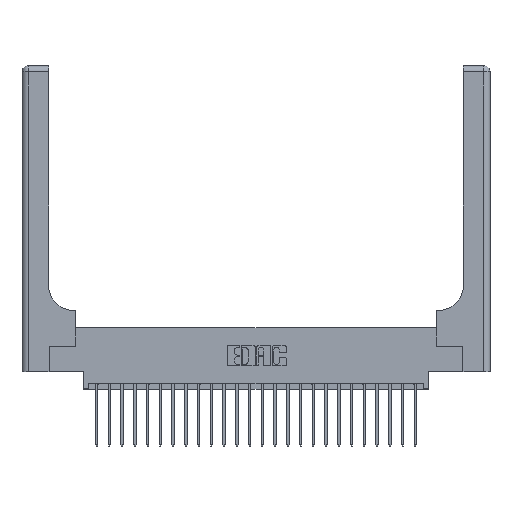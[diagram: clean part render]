
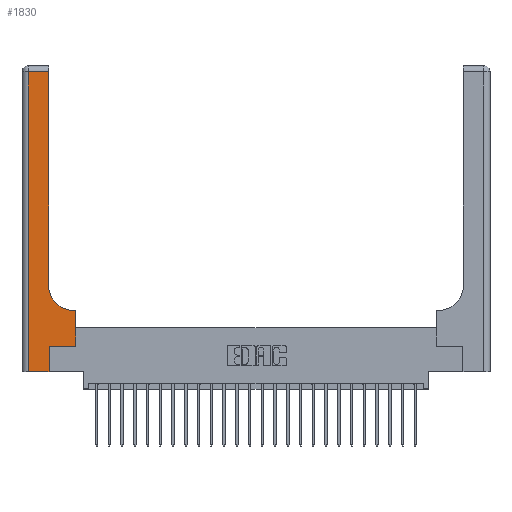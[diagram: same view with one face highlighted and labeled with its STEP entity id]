
A CAD part, top view. The second image highlights one B-rep face of the part: STEP entity #1830.
In plain terms, the highlighted planar face has unit normal (0, 0, 1).
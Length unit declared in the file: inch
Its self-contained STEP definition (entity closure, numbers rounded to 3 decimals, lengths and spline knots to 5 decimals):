
#907 = CARTESIAN_POINT ( 'NONE',  ( 0.265, 0.25, 0.37 ) ) ;
#1039 = DIRECTION ( 'NONE',  ( 1., 0., 0. ) ) ;
#1830 = ADVANCED_FACE ( 'NONE', ( #12755 ), #13224, .F. ) ;
#1839 = VECTOR ( 'NONE', #23697, 39.37008 ) ;
#2107 = CARTESIAN_POINT ( 'NONE',  ( 0., 2.94, 0.37 ) ) ;
#2507 = EDGE_CURVE ( 'NONE', #11586, #22387, #18204, .T. ) ;
#2568 = CARTESIAN_POINT ( 'NONE',  ( 0.265, 0.25, 0.37 ) ) ;
#3738 = DIRECTION ( 'NONE',  ( 0., 0., -1. ) ) ;
#3867 = DIRECTION ( 'NONE',  ( 1., 0., 0. ) ) ;
#4094 = EDGE_LOOP ( 'NONE', ( #14593, #15650, #18996, #6503, #6752, #19972, #21662, #5677, #20019 ) ) ;
#4520 = CARTESIAN_POINT ( 'NONE',  ( 0.265, 0., 0.37 ) ) ;
#5677 = ORIENTED_EDGE ( 'NONE', *, *, #22340, .T. ) ;
#5718 = EDGE_CURVE ( 'NONE', #14722, #11091, #9026, .T. ) ;
#5780 = CARTESIAN_POINT ( 'NONE',  ( 0.528, 0.25, 0.37 ) ) ;
#6503 = ORIENTED_EDGE ( 'NONE', *, *, #20031, .T. ) ;
#6692 = CARTESIAN_POINT ( 'NONE',  ( 0.528, 0.25, 0.37 ) ) ;
#6752 = ORIENTED_EDGE ( 'NONE', *, *, #20566, .T. ) ;
#7523 = CARTESIAN_POINT ( 'NONE',  ( 0.51, 0.85, 0.37 ) ) ;
#7772 = DIRECTION ( 'NONE',  ( 0., 0., -1. ) ) ;
#8217 = VERTEX_POINT ( 'NONE', #21770 ) ;
#9026 = LINE ( 'NONE', #24402, #1839 ) ;
#9103 = VECTOR ( 'NONE', #3867, 39.37008 ) ;
#9457 = DIRECTION ( 'NONE',  ( 0., 1., 0. ) ) ;
#9771 = EDGE_CURVE ( 'NONE', #24010, #11749, #13495, .T. ) ;
#10617 = DIRECTION ( 'NONE',  ( -1., 0., 0. ) ) ;
#10665 = VECTOR ( 'NONE', #10617, 39.37008 ) ;
#10922 = VECTOR ( 'NONE', #9457, 39.37008 ) ;
#11091 = VERTEX_POINT ( 'NONE', #15239 ) ;
#11327 = CARTESIAN_POINT ( 'NONE',  ( 0., 3., 0.37 ) ) ;
#11586 = VERTEX_POINT ( 'NONE', #2568 ) ;
#11749 = VERTEX_POINT ( 'NONE', #14562 ) ;
#12339 = EDGE_CURVE ( 'NONE', #11749, #8217, #13014, .T. ) ;
#12506 = CARTESIAN_POINT ( 'NONE',  ( 0.51, 0.6, 0.37 ) ) ;
#12755 = FACE_OUTER_BOUND ( 'NONE', #4094, .T. ) ;
#13014 = LINE ( 'NONE', #17042, #13514 ) ;
#13097 = VECTOR ( 'NONE', #14096, 39.37008 ) ;
#13224 = PLANE ( 'NONE',  #20413 ) ;
#13400 = DIRECTION ( 'NONE',  ( 0., 1., 0. ) ) ;
#13495 = CIRCLE ( 'NONE', #19106, 0.25 ) ;
#13514 = VECTOR ( 'NONE', #13400, 39.37008 ) ;
#13970 = LINE ( 'NONE', #2107, #13097 ) ;
#14096 = DIRECTION ( 'NONE',  ( -1., 0., 0. ) ) ;
#14511 = CARTESIAN_POINT ( 'NONE',  ( 0.528, 0.6, 0.37 ) ) ;
#14562 = CARTESIAN_POINT ( 'NONE',  ( 0.26, 0.85, 0.37 ) ) ;
#14593 = ORIENTED_EDGE ( 'NONE', *, *, #12339, .T. ) ;
#14722 = VERTEX_POINT ( 'NONE', #21581 ) ;
#15234 = LINE ( 'NONE', #19007, #9103 ) ;
#15239 = CARTESIAN_POINT ( 'NONE',  ( 0.06, 0., 0.37 ) ) ;
#15348 = DIRECTION ( 'NONE',  ( 1., 0., 0. ) ) ;
#15442 = EDGE_CURVE ( 'NONE', #22387, #16052, #20909, .T. ) ;
#15564 = CARTESIAN_POINT ( 'NONE',  ( 0.265, 0., 0.37 ) ) ;
#15650 = ORIENTED_EDGE ( 'NONE', *, *, #20215, .T. ) ;
#16052 = VERTEX_POINT ( 'NONE', #14511 ) ;
#17042 = CARTESIAN_POINT ( 'NONE',  ( 0.26, 3., 0.37 ) ) ;
#17926 = LINE ( 'NONE', #24219, #10665 ) ;
#18204 = LINE ( 'NONE', #907, #21245 ) ;
#18892 = DIRECTION ( 'NONE',  ( -1., 0., 0. ) ) ;
#18996 = ORIENTED_EDGE ( 'NONE', *, *, #5718, .T. ) ;
#19007 = CARTESIAN_POINT ( 'NONE',  ( 0., 0., 0.37 ) ) ;
#19106 = AXIS2_PLACEMENT_3D ( 'NONE', #7523, #3738, #15348 ) ;
#19468 = DIRECTION ( 'NONE',  ( 0., 1., 0. ) ) ;
#19972 = ORIENTED_EDGE ( 'NONE', *, *, #2507, .T. ) ;
#20019 = ORIENTED_EDGE ( 'NONE', *, *, #9771, .T. ) ;
#20031 = EDGE_CURVE ( 'NONE', #11091, #24439, #15234, .T. ) ;
#20215 = EDGE_CURVE ( 'NONE', #8217, #14722, #13970, .T. ) ;
#20413 = AXIS2_PLACEMENT_3D ( 'NONE', #11327, #7772, #18892 ) ;
#20566 = EDGE_CURVE ( 'NONE', #24439, #11586, #21591, .T. ) ;
#20909 = LINE ( 'NONE', #5780, #10922 ) ;
#21245 = VECTOR ( 'NONE', #1039, 39.37008 ) ;
#21581 = CARTESIAN_POINT ( 'NONE',  ( 0.06, 2.94, 0.37 ) ) ;
#21591 = LINE ( 'NONE', #15564, #21626 ) ;
#21626 = VECTOR ( 'NONE', #19468, 39.37008 ) ;
#21662 = ORIENTED_EDGE ( 'NONE', *, *, #15442, .T. ) ;
#21770 = CARTESIAN_POINT ( 'NONE',  ( 0.26, 2.94, 0.37 ) ) ;
#22340 = EDGE_CURVE ( 'NONE', #16052, #24010, #17926, .T. ) ;
#22387 = VERTEX_POINT ( 'NONE', #6692 ) ;
#23697 = DIRECTION ( 'NONE',  ( 0., -1., 0. ) ) ;
#24010 = VERTEX_POINT ( 'NONE', #12506 ) ;
#24219 = CARTESIAN_POINT ( 'NONE',  ( 0.26, 0.6, 0.37 ) ) ;
#24402 = CARTESIAN_POINT ( 'NONE',  ( 0.06, 3., 0.37 ) ) ;
#24439 = VERTEX_POINT ( 'NONE', #4520 ) ;
